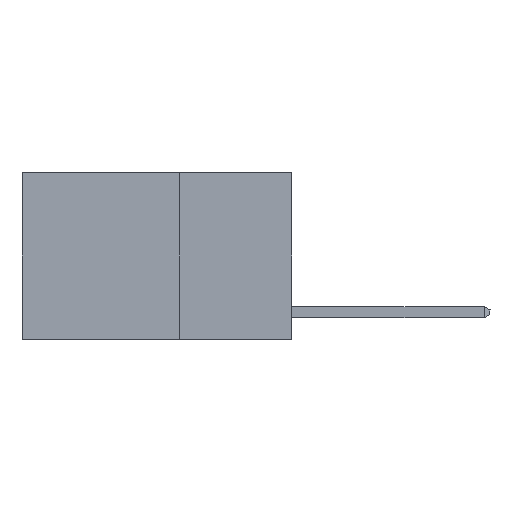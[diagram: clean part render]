
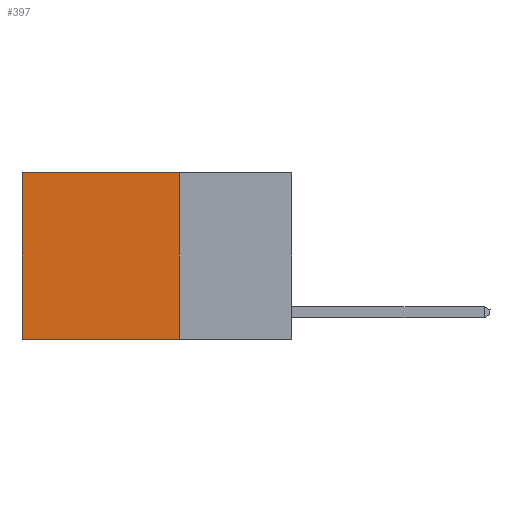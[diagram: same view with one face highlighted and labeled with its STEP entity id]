
A CAD part, left-side view. The second image highlights one B-rep face of the part: STEP entity #397.
In plain terms, the highlighted planar face has unit normal (-1, 0, 0).
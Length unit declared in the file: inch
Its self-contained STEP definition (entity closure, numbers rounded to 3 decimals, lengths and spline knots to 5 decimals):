
#12 = FACE_OUTER_BOUND ( 'NONE', #3560, .T. ) ;
#56 = CARTESIAN_POINT ( 'NONE',  ( 0.2625, 0.25, 0. ) ) ;
#66 = DIRECTION ( 'NONE',  ( 1., 0., 0. ) ) ;
#303 = LINE ( 'NONE', #5128, #5328 ) ;
#397 = ADVANCED_FACE ( 'NONE', ( #12 ), #4066, .F. ) ;
#856 = EDGE_CURVE ( 'NONE', #2200, #11066, #4561, .T. ) ;
#1058 = DIRECTION ( 'NONE',  ( 0., 0., -1. ) ) ;
#1409 = CARTESIAN_POINT ( 'NONE',  ( 0.2625, 0.25, 0. ) ) ;
#1579 = DIRECTION ( 'NONE',  ( 0., 0., -1. ) ) ;
#2200 = VERTEX_POINT ( 'NONE', #7408 ) ;
#2355 = EDGE_CURVE ( 'NONE', #6500, #11066, #303, .T. ) ;
#3425 = EDGE_CURVE ( 'NONE', #6355, #6500, #6711, .T. ) ;
#3442 = EDGE_CURVE ( 'NONE', #6355, #2200, #12955, .T. ) ;
#3537 = AXIS2_PLACEMENT_3D ( 'NONE', #11107, #66, #1058 ) ;
#3560 = EDGE_LOOP ( 'NONE', ( #10996, #4037, #9397, #9327 ) ) ;
#4037 = ORIENTED_EDGE ( 'NONE', *, *, #2355, .F. ) ;
#4043 = VECTOR ( 'NONE', #12078, 39.37008 ) ;
#4066 = PLANE ( 'NONE',  #3537 ) ;
#4561 = LINE ( 'NONE', #9607, #10550 ) ;
#5128 = CARTESIAN_POINT ( 'NONE',  ( 0.2625, 0.25, -0.37 ) ) ;
#5328 = VECTOR ( 'NONE', #11199, 39.37008 ) ;
#5517 = CARTESIAN_POINT ( 'NONE',  ( 0.2625, 0.25, -0.37 ) ) ;
#6355 = VERTEX_POINT ( 'NONE', #1409 ) ;
#6500 = VERTEX_POINT ( 'NONE', #5517 ) ;
#6711 = LINE ( 'NONE', #56, #12490 ) ;
#7408 = CARTESIAN_POINT ( 'NONE',  ( 0.2625, 0.6, 0. ) ) ;
#9190 = DIRECTION ( 'NONE',  ( 0., 0., -1. ) ) ;
#9327 = ORIENTED_EDGE ( 'NONE', *, *, #3442, .T. ) ;
#9397 = ORIENTED_EDGE ( 'NONE', *, *, #3425, .F. ) ;
#9607 = CARTESIAN_POINT ( 'NONE',  ( 0.2625, 0.6, 0. ) ) ;
#9962 = CARTESIAN_POINT ( 'NONE',  ( 0.2625, 0.6, -0.37 ) ) ;
#10550 = VECTOR ( 'NONE', #1579, 39.37008 ) ;
#10996 = ORIENTED_EDGE ( 'NONE', *, *, #856, .T. ) ;
#11066 = VERTEX_POINT ( 'NONE', #9962 ) ;
#11107 = CARTESIAN_POINT ( 'NONE',  ( 0.2625, 0.25, 0. ) ) ;
#11199 = DIRECTION ( 'NONE',  ( 0., 1., 0. ) ) ;
#11232 = CARTESIAN_POINT ( 'NONE',  ( 0.2625, 0.25, 0. ) ) ;
#12078 = DIRECTION ( 'NONE',  ( 0., 1., 0. ) ) ;
#12490 = VECTOR ( 'NONE', #9190, 39.37008 ) ;
#12955 = LINE ( 'NONE', #11232, #4043 ) ;
